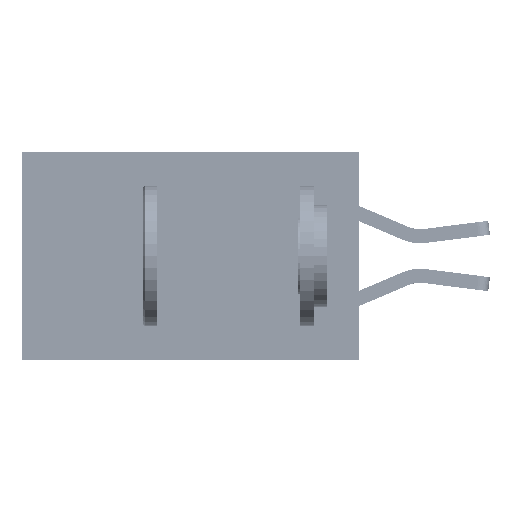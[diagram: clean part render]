
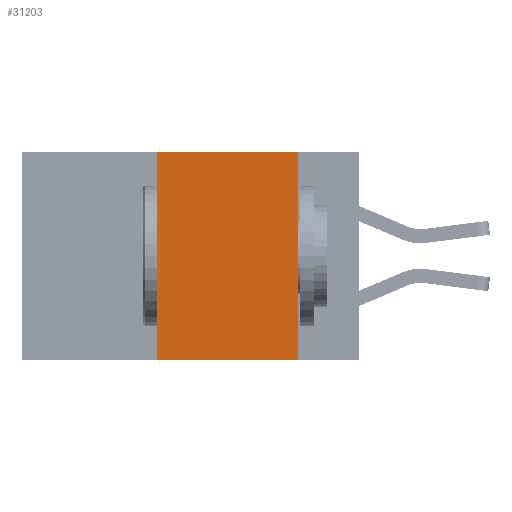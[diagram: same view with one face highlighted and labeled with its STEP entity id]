
A CAD part, left-side view. The second image highlights one B-rep face of the part: STEP entity #31203.
In plain terms, the highlighted planar face has unit normal (-1, 0, 0).
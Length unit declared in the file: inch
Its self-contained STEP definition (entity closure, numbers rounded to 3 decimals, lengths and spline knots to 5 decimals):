
#488 = VERTEX_POINT ( 'NONE', #13459 ) ;
#1372 = CARTESIAN_POINT ( 'NONE',  ( 0., 0.11, 0. ) ) ;
#2139 = EDGE_CURVE ( 'NONE', #22713, #21282, #5270, .T. ) ;
#3190 = CARTESIAN_POINT ( 'NONE',  ( 0., 0.6, -0.37 ) ) ;
#3808 = CARTESIAN_POINT ( 'NONE',  ( 0., 0.36, -0.37 ) ) ;
#4822 = ORIENTED_EDGE ( 'NONE', *, *, #2139, .F. ) ;
#4829 = EDGE_CURVE ( 'NONE', #488, #22713, #27255, .T. ) ;
#5270 = LINE ( 'NONE', #19741, #7674 ) ;
#6020 = VECTOR ( 'NONE', #31383, 39.37008 ) ;
#6241 = CARTESIAN_POINT ( 'NONE',  ( 0., 0.36, 0. ) ) ;
#6801 = DIRECTION ( 'NONE',  ( 0., 0., -1. ) ) ;
#7215 = DIRECTION ( 'NONE',  ( 0., 0., -1. ) ) ;
#7223 = CARTESIAN_POINT ( 'NONE',  ( 0., 0.6, 0. ) ) ;
#7674 = VECTOR ( 'NONE', #7215, 39.37008 ) ;
#7958 = VECTOR ( 'NONE', #34462, 39.37008 ) ;
#9406 = EDGE_CURVE ( 'NONE', #27238, #21282, #23420, .T. ) ;
#10191 = PLANE ( 'NONE',  #26457 ) ;
#11941 = CARTESIAN_POINT ( 'NONE',  ( 0., 0.6, 0. ) ) ;
#13459 = CARTESIAN_POINT ( 'NONE',  ( 0., 0.36, 0. ) ) ;
#16391 = DIRECTION ( 'NONE',  ( 1., 0., 0. ) ) ;
#18814 = EDGE_LOOP ( 'NONE', ( #4822, #29185, #20365, #30923 ) ) ;
#19464 = EDGE_CURVE ( 'NONE', #27238, #488, #24685, .T. ) ;
#19741 = CARTESIAN_POINT ( 'NONE',  ( 0., 0.11, 0. ) ) ;
#20365 = ORIENTED_EDGE ( 'NONE', *, *, #19464, .F. ) ;
#21282 = VERTEX_POINT ( 'NONE', #24139 ) ;
#22713 = VERTEX_POINT ( 'NONE', #1372 ) ;
#23420 = LINE ( 'NONE', #3190, #6020 ) ;
#24139 = CARTESIAN_POINT ( 'NONE',  ( 0., 0.11, -0.37 ) ) ;
#24685 = LINE ( 'NONE', #6241, #37251 ) ;
#26457 = AXIS2_PLACEMENT_3D ( 'NONE', #7223, #16391, #6801 ) ;
#27238 = VERTEX_POINT ( 'NONE', #3808 ) ;
#27255 = LINE ( 'NONE', #11941, #7958 ) ;
#29185 = ORIENTED_EDGE ( 'NONE', *, *, #4829, .F. ) ;
#30923 = ORIENTED_EDGE ( 'NONE', *, *, #9406, .T. ) ;
#31203 = ADVANCED_FACE ( 'NONE', ( #34680 ), #10191, .F. ) ;
#31383 = DIRECTION ( 'NONE',  ( 0., -1., 0. ) ) ;
#34462 = DIRECTION ( 'NONE',  ( 0., -1., 0. ) ) ;
#34680 = FACE_OUTER_BOUND ( 'NONE', #18814, .T. ) ;
#36752 = DIRECTION ( 'NONE',  ( 0., 0., 1. ) ) ;
#37251 = VECTOR ( 'NONE', #36752, 39.37008 ) ;
